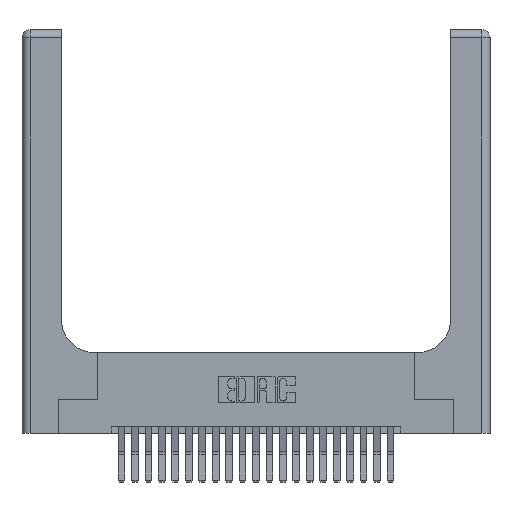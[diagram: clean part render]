
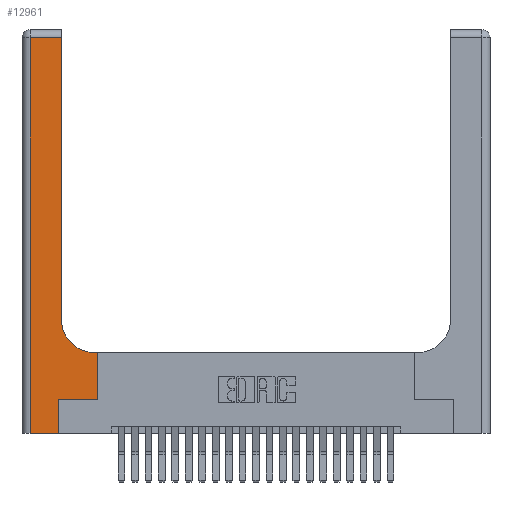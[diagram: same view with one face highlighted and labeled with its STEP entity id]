
A CAD part, top view. The second image highlights one B-rep face of the part: STEP entity #12961.
In plain terms, the highlighted planar face has unit normal (0, 0, 1).
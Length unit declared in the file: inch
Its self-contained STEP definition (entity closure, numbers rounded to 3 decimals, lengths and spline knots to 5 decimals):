
#88 = DIRECTION ( 'NONE',  ( 0., 1., 0. ) ) ;
#758 = DIRECTION ( 'NONE',  ( -1., 0., 0. ) ) ;
#1229 = ORIENTED_EDGE ( 'NONE', *, *, #22242, .T. ) ;
#1365 = VERTEX_POINT ( 'NONE', #2135 ) ;
#1444 = VERTEX_POINT ( 'NONE', #11933 ) ;
#1550 = FACE_OUTER_BOUND ( 'NONE', #1743, .T. ) ;
#1743 = EDGE_LOOP ( 'NONE', ( #3115, #20034, #23147, #15236, #6361, #1229, #18204, #11070, #12186 ) ) ;
#1824 = VERTEX_POINT ( 'NONE', #3954 ) ;
#2135 = CARTESIAN_POINT ( 'NONE',  ( 0.2915, 2.94, 0.37 ) ) ;
#2271 = DIRECTION ( 'NONE',  ( 0., 1., 0. ) ) ;
#2429 = EDGE_CURVE ( 'NONE', #10785, #1824, #23724, .T. ) ;
#2441 = CARTESIAN_POINT ( 'NONE',  ( 0.269, 0., 0.37 ) ) ;
#2698 = DIRECTION ( 'NONE',  ( 1., 0., 0. ) ) ;
#3115 = ORIENTED_EDGE ( 'NONE', *, *, #5142, .T. ) ;
#3250 = DIRECTION ( 'NONE',  ( 0., -1., 0. ) ) ;
#3291 = DIRECTION ( 'NONE',  ( -1., 0., 0. ) ) ;
#3316 = CARTESIAN_POINT ( 'NONE',  ( 0.5415, 0.85, 0.37 ) ) ;
#3353 = DIRECTION ( 'NONE',  ( 0., 1., 0. ) ) ;
#3414 = DIRECTION ( 'NONE',  ( -1., 0., 0. ) ) ;
#3748 = EDGE_CURVE ( 'NONE', #1365, #14247, #10867, .T. ) ;
#3954 = CARTESIAN_POINT ( 'NONE',  ( 0.2915, 0.85, 0.37 ) ) ;
#3994 = CARTESIAN_POINT ( 'NONE',  ( 0.269, 0.25, 0.37 ) ) ;
#4372 = VECTOR ( 'NONE', #3250, 39.37008 ) ;
#5142 = EDGE_CURVE ( 'NONE', #1824, #1365, #22161, .T. ) ;
#5217 = DIRECTION ( 'NONE',  ( 1., 0., 0. ) ) ;
#5369 = LINE ( 'NONE', #10337, #11628 ) ;
#5486 = CARTESIAN_POINT ( 'NONE',  ( 0.2915, 3., 0.37 ) ) ;
#5551 = CARTESIAN_POINT ( 'NONE',  ( 0., 3., 0.37 ) ) ;
#5658 = EDGE_CURVE ( 'NONE', #20721, #1444, #13019, .T. ) ;
#5848 = DIRECTION ( 'NONE',  ( 1., 0., 0. ) ) ;
#6313 = EDGE_CURVE ( 'NONE', #14247, #20721, #8232, .T. ) ;
#6361 = ORIENTED_EDGE ( 'NONE', *, *, #7091, .T. ) ;
#7091 = EDGE_CURVE ( 'NONE', #1444, #9977, #12093, .T. ) ;
#7163 = VERTEX_POINT ( 'NONE', #23347 ) ;
#7283 = PLANE ( 'NONE',  #10830 ) ;
#7840 = CARTESIAN_POINT ( 'NONE',  ( 0.06, 2.94, 0.37 ) ) ;
#8232 = LINE ( 'NONE', #16698, #4372 ) ;
#8247 = CARTESIAN_POINT ( 'NONE',  ( 0.5415, 0.6, 0.37 ) ) ;
#8600 = CARTESIAN_POINT ( 'NONE',  ( 0.06, 0., 0.37 ) ) ;
#8936 = VERTEX_POINT ( 'NONE', #17445 ) ;
#9977 = VERTEX_POINT ( 'NONE', #3994 ) ;
#10045 = EDGE_CURVE ( 'NONE', #7163, #8936, #18474, .T. ) ;
#10337 = CARTESIAN_POINT ( 'NONE',  ( 0.269, 0.25, 0.37 ) ) ;
#10785 = VERTEX_POINT ( 'NONE', #8247 ) ;
#10830 = AXIS2_PLACEMENT_3D ( 'NONE', #5551, #11202, #3414 ) ;
#10867 = LINE ( 'NONE', #14702, #15914 ) ;
#11070 = ORIENTED_EDGE ( 'NONE', *, *, #14403, .T. ) ;
#11202 = DIRECTION ( 'NONE',  ( 0., 0., -1. ) ) ;
#11551 = CARTESIAN_POINT ( 'NONE',  ( 0.5585, 0.25, 0.37 ) ) ;
#11628 = VECTOR ( 'NONE', #2698, 39.37008 ) ;
#11933 = CARTESIAN_POINT ( 'NONE',  ( 0.269, 0., 0.37 ) ) ;
#12093 = LINE ( 'NONE', #2441, #16554 ) ;
#12186 = ORIENTED_EDGE ( 'NONE', *, *, #2429, .T. ) ;
#12527 = VECTOR ( 'NONE', #88, 39.37008 ) ;
#12961 = ADVANCED_FACE ( 'NONE', ( #1550 ), #7283, .F. ) ;
#13019 = LINE ( 'NONE', #15264, #13313 ) ;
#13313 = VECTOR ( 'NONE', #5848, 39.37008 ) ;
#14247 = VERTEX_POINT ( 'NONE', #7840 ) ;
#14268 = VECTOR ( 'NONE', #758, 39.37008 ) ;
#14403 = EDGE_CURVE ( 'NONE', #8936, #10785, #19305, .T. ) ;
#14702 = CARTESIAN_POINT ( 'NONE',  ( 0., 2.94, 0.37 ) ) ;
#15236 = ORIENTED_EDGE ( 'NONE', *, *, #5658, .T. ) ;
#15264 = CARTESIAN_POINT ( 'NONE',  ( 0., 0., 0.37 ) ) ;
#15914 = VECTOR ( 'NONE', #3291, 39.37008 ) ;
#16554 = VECTOR ( 'NONE', #2271, 39.37008 ) ;
#16698 = CARTESIAN_POINT ( 'NONE',  ( 0.06, 3., 0.37 ) ) ;
#17095 = VECTOR ( 'NONE', #3353, 39.37008 ) ;
#17445 = CARTESIAN_POINT ( 'NONE',  ( 0.5585, 0.6, 0.37 ) ) ;
#18204 = ORIENTED_EDGE ( 'NONE', *, *, #10045, .T. ) ;
#18278 = DIRECTION ( 'NONE',  ( 0., 0., -1. ) ) ;
#18474 = LINE ( 'NONE', #11551, #12527 ) ;
#19305 = LINE ( 'NONE', #23512, #14268 ) ;
#20034 = ORIENTED_EDGE ( 'NONE', *, *, #3748, .T. ) ;
#20721 = VERTEX_POINT ( 'NONE', #8600 ) ;
#22161 = LINE ( 'NONE', #5486, #17095 ) ;
#22242 = EDGE_CURVE ( 'NONE', #9977, #7163, #5369, .T. ) ;
#22426 = AXIS2_PLACEMENT_3D ( 'NONE', #3316, #18278, #5217 ) ;
#23147 = ORIENTED_EDGE ( 'NONE', *, *, #6313, .T. ) ;
#23347 = CARTESIAN_POINT ( 'NONE',  ( 0.5585, 0.25, 0.37 ) ) ;
#23512 = CARTESIAN_POINT ( 'NONE',  ( 0.2915, 0.6, 0.37 ) ) ;
#23724 = CIRCLE ( 'NONE', #22426, 0.25 ) ;
